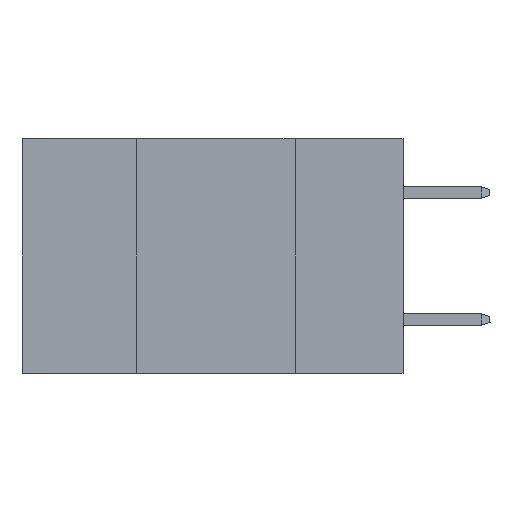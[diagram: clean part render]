
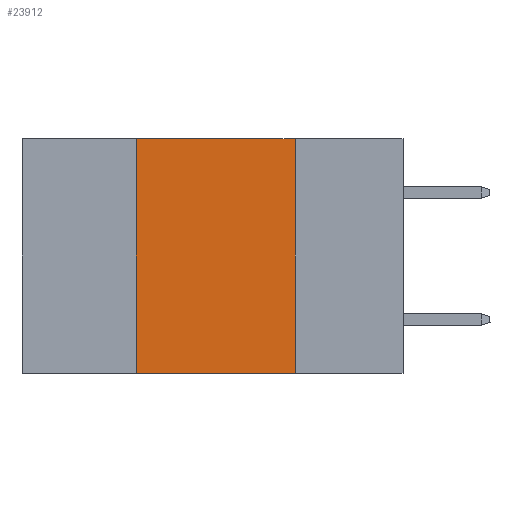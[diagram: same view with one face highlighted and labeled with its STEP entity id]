
A CAD part, left-side view. The second image highlights one B-rep face of the part: STEP entity #23912.
In plain terms, the highlighted planar face has unit normal (-1, 0, 0).
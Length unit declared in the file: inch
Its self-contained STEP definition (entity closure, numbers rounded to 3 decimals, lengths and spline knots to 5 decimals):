
#726 = EDGE_CURVE ( 'NONE', #23727, #10765, #13120, .T. ) ;
#1347 = DIRECTION ( 'NONE',  ( 0., 0., -1. ) ) ;
#1777 = VECTOR ( 'NONE', #21951, 39.37008 ) ;
#2258 = AXIS2_PLACEMENT_3D ( 'NONE', #3290, #14844, #18713 ) ;
#2525 = LINE ( 'NONE', #24085, #1777 ) ;
#3137 = CARTESIAN_POINT ( 'NONE',  ( 0., 0.6, -0.37 ) ) ;
#3290 = CARTESIAN_POINT ( 'NONE',  ( 0., 0.6, 0. ) ) ;
#3401 = VERTEX_POINT ( 'NONE', #9850 ) ;
#5208 = ORIENTED_EDGE ( 'NONE', *, *, #20139, .F. ) ;
#5464 = CARTESIAN_POINT ( 'NONE',  ( 0., 0.6, 0. ) ) ;
#6051 = EDGE_LOOP ( 'NONE', ( #5208, #20734, #16020, #12368 ) ) ;
#9141 = LINE ( 'NONE', #3137, #13036 ) ;
#9225 = DIRECTION ( 'NONE',  ( 0., -1., 0. ) ) ;
#9850 = CARTESIAN_POINT ( 'NONE',  ( 0., 0.42, -0.37 ) ) ;
#10040 = VECTOR ( 'NONE', #9225, 39.37008 ) ;
#10765 = VERTEX_POINT ( 'NONE', #15553 ) ;
#10817 = PLANE ( 'NONE',  #2258 ) ;
#10876 = LINE ( 'NONE', #18517, #24216 ) ;
#11281 = DIRECTION ( 'NONE',  ( 0., -1., 0. ) ) ;
#12368 = ORIENTED_EDGE ( 'NONE', *, *, #21046, .T. ) ;
#13036 = VECTOR ( 'NONE', #11281, 39.37008 ) ;
#13120 = LINE ( 'NONE', #5464, #10040 ) ;
#13795 = CARTESIAN_POINT ( 'NONE',  ( 0., 0.17, -0.37 ) ) ;
#14844 = DIRECTION ( 'NONE',  ( 1., 0., 0. ) ) ;
#15553 = CARTESIAN_POINT ( 'NONE',  ( 0., 0.17, 0. ) ) ;
#16020 = ORIENTED_EDGE ( 'NONE', *, *, #19166, .F. ) ;
#16611 = VERTEX_POINT ( 'NONE', #13795 ) ;
#18517 = CARTESIAN_POINT ( 'NONE',  ( 0., 0.17, 0. ) ) ;
#18713 = DIRECTION ( 'NONE',  ( 0., 0., -1. ) ) ;
#19166 = EDGE_CURVE ( 'NONE', #3401, #23727, #2525, .T. ) ;
#20139 = EDGE_CURVE ( 'NONE', #10765, #16611, #10876, .T. ) ;
#20578 = FACE_OUTER_BOUND ( 'NONE', #6051, .T. ) ;
#20734 = ORIENTED_EDGE ( 'NONE', *, *, #726, .F. ) ;
#21046 = EDGE_CURVE ( 'NONE', #3401, #16611, #9141, .T. ) ;
#21951 = DIRECTION ( 'NONE',  ( 0., 0., 1. ) ) ;
#22718 = CARTESIAN_POINT ( 'NONE',  ( 0., 0.42, 0. ) ) ;
#23727 = VERTEX_POINT ( 'NONE', #22718 ) ;
#23912 = ADVANCED_FACE ( 'NONE', ( #20578 ), #10817, .F. ) ;
#24085 = CARTESIAN_POINT ( 'NONE',  ( 0., 0.42, 0. ) ) ;
#24216 = VECTOR ( 'NONE', #1347, 39.37008 ) ;
